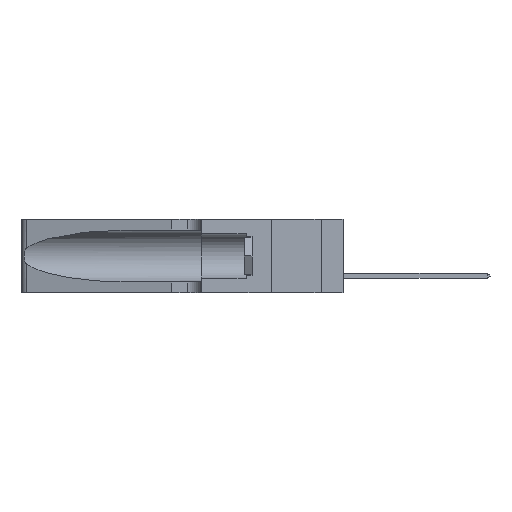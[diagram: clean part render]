
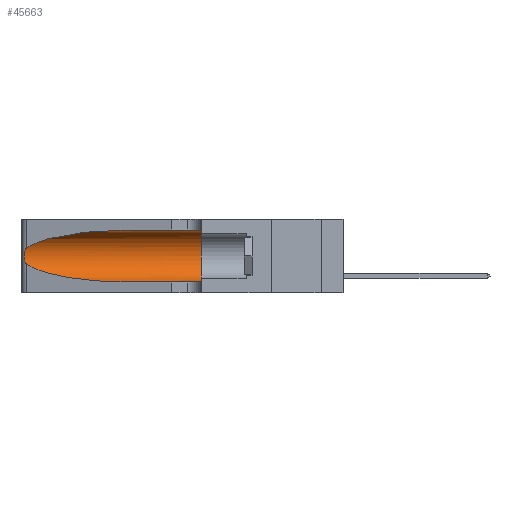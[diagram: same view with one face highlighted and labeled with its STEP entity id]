
A CAD part, left-side view. The second image highlights one B-rep face of the part: STEP entity #45663.
In plain terms, the highlighted cylindrical face has radius 3.308 mm (diameter 6.617 mm), a partial arc.
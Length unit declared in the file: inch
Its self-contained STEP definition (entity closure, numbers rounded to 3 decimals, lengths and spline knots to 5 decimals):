
#20 = EDGE_CURVE ( 'NONE', #4184, #12813, #29520, .T. ) ;
#463 = CIRCLE ( 'NONE', #15910, 0.13025 ) ;
#951 = CARTESIAN_POINT ( 'NONE',  ( 0.25487, 1.22718, 0.22369 ) ) ;
#1292 = DIRECTION ( 'NONE',  ( 0., 1., 0. ) ) ;
#1945 = AXIS2_PLACEMENT_3D ( 'NONE', #15689, #23383, #38652 ) ;
#3001 = CARTESIAN_POINT ( 'NONE',  ( 0.25487, 1.22718, 0.14631 ) ) ;
#4184 = VERTEX_POINT ( 'NONE', #3001 ) ;
#4314 = CARTESIAN_POINT ( 'NONE',  ( 0.25854, 1.2359, 0.20912 ) ) ;
#6549 = CARTESIAN_POINT ( 'NONE',  ( 0.25487, 1.22718, 0.14631 ) ) ;
#9310 = CARTESIAN_POINT ( 'NONE',  ( 0.1305, 1.61858, 0.05475 ) ) ;
#9315 = LINE ( 'NONE', #9310, #18527 ) ;
#10899 = CARTESIAN_POINT ( 'NONE',  ( 0.1305, 0.35, 0.05475 ) ) ;
#12287 = DIRECTION ( 'NONE',  ( 0., 0., 1. ) ) ;
#12700 = DIRECTION ( 'NONE',  ( 0., -1., 0. ) ) ;
#12813 = VERTEX_POINT ( 'NONE', #42521 ) ;
#13647 = CARTESIAN_POINT ( 'NONE',  ( 0.25555, 1.22993, 0.14849 ) ) ;
#14694 = EDGE_CURVE ( 'NONE', #46107, #41564, #463, .T. ) ;
#14863 = VERTEX_POINT ( 'NONE', #26673 ) ;
#15689 = CARTESIAN_POINT ( 'NONE',  ( 0.1305, 1.61858, 0.185 ) ) ;
#15910 = AXIS2_PLACEMENT_3D ( 'NONE', #35076, #1292, #12287 ) ;
#15982 = CARTESIAN_POINT ( 'NONE',  ( 0.25639, 1.23184, 0.21858 ) ) ;
#16167 = VECTOR ( 'NONE', #12700, 39.37008 ) ;
#16682 = ORIENTED_EDGE ( 'NONE', *, *, #14694, .F. ) ;
#16739 = CARTESIAN_POINT ( 'NONE',  ( 0.26018, 1.23835, 0.19895 ) ) ;
#17911 = LINE ( 'NONE', #31107, #16167 ) ;
#18527 = VECTOR ( 'NONE', #46531, 39.37008 ) ;
#19519 = FACE_OUTER_BOUND ( 'NONE', #40698, .T. ) ;
#20301 = ORIENTED_EDGE ( 'NONE', *, *, #29220, .T. ) ;
#20535 = CARTESIAN_POINT ( 'NONE',  ( 0.25789, 1.23486, 0.15765 ) ) ;
#21184 = CARTESIAN_POINT ( 'NONE',  ( 0.25856, 1.23593, 0.16098 ) ) ;
#23383 = DIRECTION ( 'NONE',  ( 0., -1., 0. ) ) ;
#24247 = CARTESIAN_POINT ( 'NONE',  ( 0.18966, 0.96281, 0.31525 ) ) ;
#25107 = ORIENTED_EDGE ( 'NONE', *, *, #29684, .T. ) ;
#26673 = CARTESIAN_POINT ( 'NONE',  ( 0.25487, 1.22718, 0.22369 ) ) ;
#27308 = CARTESIAN_POINT ( 'NONE',  ( 0.2373, 1.15595, 0.28018 ) ) ;
#27475 = CARTESIAN_POINT ( 'NONE',  ( 0.25487, 1.22718, 0.22369 ) ) ;
#28198 = CARTESIAN_POINT ( 'NONE',  ( 0.25487, 1.22718, 0.14631 ) ) ;
#29220 = EDGE_CURVE ( 'NONE', #32537, #14863, #34524, .T. ) ;
#29262 = ORIENTED_EDGE ( 'NONE', *, *, #35789, .F. ) ;
#29487 = ORIENTED_EDGE ( 'NONE', *, *, #34425, .T. ) ;
#29520 =( BOUNDED_CURVE ( )  B_SPLINE_CURVE ( 3, ( #6549, #35842, #32752, #43312 ),
 .UNSPECIFIED., .F., .F. ) 
 B_SPLINE_CURVE_WITH_KNOTS ( ( 4, 4 ),
 ( 3.44316, 4.71239 ),
 .UNSPECIFIED. ) 
 CURVE ( )  GEOMETRIC_REPRESENTATION_ITEM ( )  RATIONAL_B_SPLINE_CURVE ( ( 1., 0.87, 0.87, 1. ) ) 
 REPRESENTATION_ITEM ( '' )  );
#29684 = EDGE_CURVE ( 'NONE', #14863, #4184, #30667, .T. ) ;
#30123 = CARTESIAN_POINT ( 'NONE',  ( 0.1305, 0.72297, 0.31525 ) ) ;
#30667 = B_SPLINE_CURVE_WITH_KNOTS ( 'NONE', 3,
 ( #951, #34400, #15982, #33915, #4314, #16739, #46707, #46538, #35325, #21184, #20535, #31591, #13647, #28198 ),
 .UNSPECIFIED., .F., .F.,
 ( 4, 2, 2, 2, 2, 2, 4 ),
 ( 0., 0.00027, 0.00053, 0.00107, 0.0016, 0.00187, 0.00214 ),
 .UNSPECIFIED. ) ;
#31107 = CARTESIAN_POINT ( 'NONE',  ( 0.1305, 1.61858, 0.31525 ) ) ;
#31591 = CARTESIAN_POINT ( 'NONE',  ( 0.25639, 1.23186, 0.15144 ) ) ;
#32537 = VERTEX_POINT ( 'NONE', #41576 ) ;
#32752 = CARTESIAN_POINT ( 'NONE',  ( 0.18966, 0.96281, 0.05475 ) ) ;
#33915 = CARTESIAN_POINT ( 'NONE',  ( 0.25787, 1.23484, 0.2124 ) ) ;
#34400 = CARTESIAN_POINT ( 'NONE',  ( 0.25555, 1.22994, 0.2215 ) ) ;
#34425 = EDGE_CURVE ( 'NONE', #12813, #41564, #9315, .T. ) ;
#34524 =( BOUNDED_CURVE ( )  B_SPLINE_CURVE ( 3, ( #30123, #24247, #27308, #27475 ),
 .UNSPECIFIED., .F., .T. ) 
 B_SPLINE_CURVE_WITH_KNOTS ( ( 4, 4 ),
 ( 1.5708, 2.84003 ),
 .UNSPECIFIED. ) 
 CURVE ( )  GEOMETRIC_REPRESENTATION_ITEM ( )  RATIONAL_B_SPLINE_CURVE ( ( 1., 0.87, 0.87, 1. ) ) 
 REPRESENTATION_ITEM ( '' )  );
#35076 = CARTESIAN_POINT ( 'NONE',  ( 0.1305, 0.35, 0.185 ) ) ;
#35325 = CARTESIAN_POINT ( 'NONE',  ( 0.26017, 1.23833, 0.17102 ) ) ;
#35789 = EDGE_CURVE ( 'NONE', #32537, #46107, #17911, .T. ) ;
#35842 = CARTESIAN_POINT ( 'NONE',  ( 0.2373, 1.15595, 0.08982 ) ) ;
#38652 = DIRECTION ( 'NONE',  ( 0., 0., -1. ) ) ;
#39787 = ORIENTED_EDGE ( 'NONE', *, *, #20, .T. ) ;
#40698 = EDGE_LOOP ( 'NONE', ( #20301, #25107, #39787, #29487, #16682, #29262 ) ) ;
#41564 = VERTEX_POINT ( 'NONE', #10899 ) ;
#41576 = CARTESIAN_POINT ( 'NONE',  ( 0.1305, 0.72297, 0.31525 ) ) ;
#41618 = CYLINDRICAL_SURFACE ( 'NONE', #1945, 0.13025 ) ;
#42521 = CARTESIAN_POINT ( 'NONE',  ( 0.1305, 0.72297, 0.05475 ) ) ;
#43312 = CARTESIAN_POINT ( 'NONE',  ( 0.1305, 0.72297, 0.05475 ) ) ;
#45448 = CARTESIAN_POINT ( 'NONE',  ( 0.1305, 0.35, 0.31525 ) ) ;
#45663 = ADVANCED_FACE ( 'NONE', ( #19519 ), #41618, .F. ) ;
#46107 = VERTEX_POINT ( 'NONE', #45448 ) ;
#46531 = DIRECTION ( 'NONE',  ( 0., -1., 0. ) ) ;
#46538 = CARTESIAN_POINT ( 'NONE',  ( 0.26075, 1.23896, 0.178 ) ) ;
#46707 = CARTESIAN_POINT ( 'NONE',  ( 0.26075, 1.23896, 0.19203 ) ) ;
